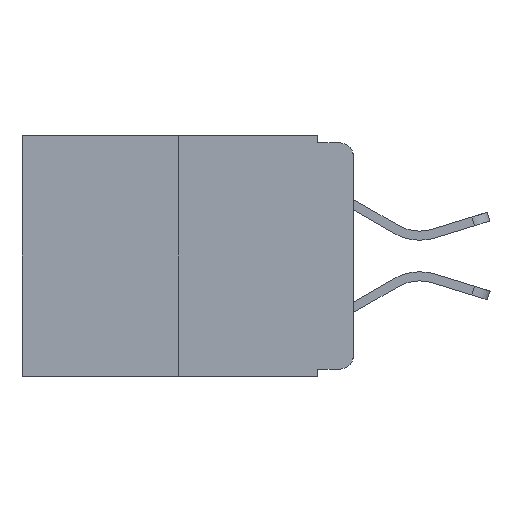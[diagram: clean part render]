
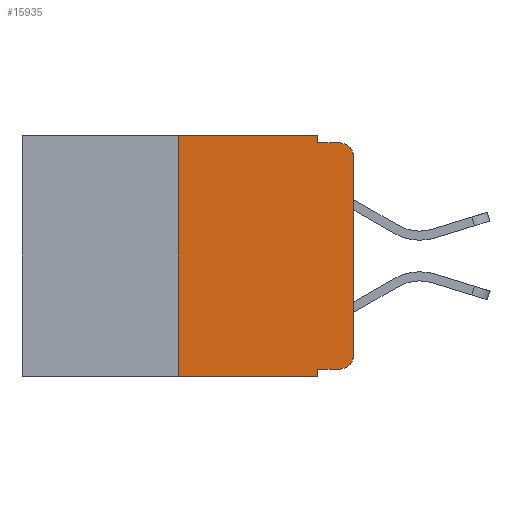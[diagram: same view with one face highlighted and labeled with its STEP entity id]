
A CAD part, left-side view. The second image highlights one B-rep face of the part: STEP entity #15935.
In plain terms, the highlighted planar face has unit normal (-1, 0, 0).
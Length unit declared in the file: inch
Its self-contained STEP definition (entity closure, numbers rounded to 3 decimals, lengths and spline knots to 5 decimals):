
#294 = CARTESIAN_POINT ( 'NONE',  ( 0., 0.051, -0.333 ) ) ;
#400 = VECTOR ( 'NONE', #10539, 39.37008 ) ;
#865 = EDGE_CURVE ( 'NONE', #15605, #11116, #6117, .T. ) ;
#1039 = LINE ( 'NONE', #8355, #7173 ) ;
#1215 = DIRECTION ( 'NONE',  ( 0., 0., 1. ) ) ;
#1316 = AXIS2_PLACEMENT_3D ( 'NONE', #6668, #11313, #2553 ) ;
#1651 = VERTEX_POINT ( 'NONE', #7602 ) ;
#1669 = CARTESIAN_POINT ( 'NONE',  ( 0., 0.25, 0. ) ) ;
#2003 = ORIENTED_EDGE ( 'NONE', *, *, #8652, .F. ) ;
#2007 = CARTESIAN_POINT ( 'NONE',  ( 0., 0.02, -0.03 ) ) ;
#2306 = DIRECTION ( 'NONE',  ( 0., -1., 0. ) ) ;
#2553 = DIRECTION ( 'NONE',  ( 0., 0., -1. ) ) ;
#2611 = EDGE_CURVE ( 'NONE', #11900, #15605, #6911, .T. ) ;
#2836 = LINE ( 'NONE', #11430, #16879 ) ;
#3022 = CARTESIAN_POINT ( 'NONE',  ( 0., 0., 0. ) ) ;
#3719 = ORIENTED_EDGE ( 'NONE', *, *, #9662, .F. ) ;
#4295 = DIRECTION ( 'NONE',  ( 0., -1., 0. ) ) ;
#4347 = EDGE_CURVE ( 'NONE', #10355, #1651, #14121, .T. ) ;
#4500 = VECTOR ( 'NONE', #1215, 39.37008 ) ;
#4568 = LINE ( 'NONE', #8996, #400 ) ;
#5197 = DIRECTION ( 'NONE',  ( 0., 0., 1. ) ) ;
#5552 = DIRECTION ( 'NONE',  ( 0., 0., -1. ) ) ;
#5730 = LINE ( 'NONE', #17534, #10146 ) ;
#5777 = EDGE_CURVE ( 'NONE', #10741, #11241, #5730, .T. ) ;
#6117 = CIRCLE ( 'NONE', #16936, 0.02 ) ;
#6533 = EDGE_CURVE ( 'NONE', #15993, #1651, #16504, .T. ) ;
#6590 = CARTESIAN_POINT ( 'NONE',  ( 0., 0.02, -0.313 ) ) ;
#6668 = CARTESIAN_POINT ( 'NONE',  ( 0., 0.473, 0. ) ) ;
#6734 = LINE ( 'NONE', #15803, #13679 ) ;
#6768 = PLANE ( 'NONE',  #1316 ) ;
#6911 = LINE ( 'NONE', #17268, #8942 ) ;
#7173 = VECTOR ( 'NONE', #2306, 39.37008 ) ;
#7587 = ORIENTED_EDGE ( 'NONE', *, *, #16901, .F. ) ;
#7602 = CARTESIAN_POINT ( 'NONE',  ( 0., 0.02, -0.01 ) ) ;
#7891 = EDGE_CURVE ( 'NONE', #18049, #15824, #1039, .T. ) ;
#8130 = CARTESIAN_POINT ( 'NONE',  ( 0., 0.051, -0.343 ) ) ;
#8355 = CARTESIAN_POINT ( 'NONE',  ( 0., 0.473, -0.343 ) ) ;
#8652 = EDGE_CURVE ( 'NONE', #18049, #10741, #6734, .T. ) ;
#8942 = VECTOR ( 'NONE', #12995, 39.37008 ) ;
#8996 = CARTESIAN_POINT ( 'NONE',  ( 0., 0.051, 0. ) ) ;
#9662 = EDGE_CURVE ( 'NONE', #11900, #15824, #2836, .T. ) ;
#9881 = ORIENTED_EDGE ( 'NONE', *, *, #7891, .T. ) ;
#9899 = ORIENTED_EDGE ( 'NONE', *, *, #2611, .T. ) ;
#9979 = CARTESIAN_POINT ( 'NONE',  ( 0., 0.25, -0.343 ) ) ;
#10015 = ORIENTED_EDGE ( 'NONE', *, *, #6533, .F. ) ;
#10146 = VECTOR ( 'NONE', #4295, 39.37008 ) ;
#10355 = VERTEX_POINT ( 'NONE', #18428 ) ;
#10539 = DIRECTION ( 'NONE',  ( 0., 0., -1. ) ) ;
#10741 = VERTEX_POINT ( 'NONE', #1669 ) ;
#11116 = VERTEX_POINT ( 'NONE', #18305 ) ;
#11241 = VERTEX_POINT ( 'NONE', #16039 ) ;
#11313 = DIRECTION ( 'NONE',  ( 1., 0., 0. ) ) ;
#11430 = CARTESIAN_POINT ( 'NONE',  ( 0., 0.051, 0. ) ) ;
#11527 = LINE ( 'NONE', #3022, #4500 ) ;
#11900 = VERTEX_POINT ( 'NONE', #294 ) ;
#12059 = CARTESIAN_POINT ( 'NONE',  ( 0., 0.051, -0.01 ) ) ;
#12681 = DIRECTION ( 'NONE',  ( -1., 0., 0. ) ) ;
#12700 = EDGE_CURVE ( 'NONE', #11116, #10355, #11527, .T. ) ;
#12995 = DIRECTION ( 'NONE',  ( 0., -1., 0. ) ) ;
#13608 = CARTESIAN_POINT ( 'NONE',  ( 0., 0.051, -0.01 ) ) ;
#13679 = VECTOR ( 'NONE', #5197, 39.37008 ) ;
#13752 = DIRECTION ( 'NONE',  ( -1., 0., 0. ) ) ;
#14121 = CIRCLE ( 'NONE', #15668, 0.02 ) ;
#14202 = ORIENTED_EDGE ( 'NONE', *, *, #12700, .T. ) ;
#14303 = DIRECTION ( 'NONE',  ( 0., 0., -1. ) ) ;
#14853 = ORIENTED_EDGE ( 'NONE', *, *, #865, .T. ) ;
#15357 = DIRECTION ( 'NONE',  ( 0., -1., 0. ) ) ;
#15461 = VECTOR ( 'NONE', #15357, 39.37008 ) ;
#15605 = VERTEX_POINT ( 'NONE', #15766 ) ;
#15668 = AXIS2_PLACEMENT_3D ( 'NONE', #2007, #13752, #5552 ) ;
#15766 = CARTESIAN_POINT ( 'NONE',  ( 0., 0.02, -0.333 ) ) ;
#15803 = CARTESIAN_POINT ( 'NONE',  ( 0., 0.25, 0. ) ) ;
#15824 = VERTEX_POINT ( 'NONE', #8130 ) ;
#15838 = FACE_OUTER_BOUND ( 'NONE', #17122, .T. ) ;
#15935 = ADVANCED_FACE ( 'NONE', ( #15838 ), #6768, .F. ) ;
#15993 = VERTEX_POINT ( 'NONE', #12059 ) ;
#16039 = CARTESIAN_POINT ( 'NONE',  ( 0., 0.051, 0. ) ) ;
#16139 = ORIENTED_EDGE ( 'NONE', *, *, #5777, .F. ) ;
#16504 = LINE ( 'NONE', #13608, #15461 ) ;
#16879 = VECTOR ( 'NONE', #17322, 39.37008 ) ;
#16901 = EDGE_CURVE ( 'NONE', #11241, #15993, #4568, .T. ) ;
#16924 = ORIENTED_EDGE ( 'NONE', *, *, #4347, .T. ) ;
#16936 = AXIS2_PLACEMENT_3D ( 'NONE', #6590, #12681, #14303 ) ;
#17122 = EDGE_LOOP ( 'NONE', ( #14202, #16924, #10015, #7587, #16139, #2003, #9881, #3719, #9899, #14853 ) ) ;
#17268 = CARTESIAN_POINT ( 'NONE',  ( 0., 0.051, -0.333 ) ) ;
#17322 = DIRECTION ( 'NONE',  ( 0., 0., -1. ) ) ;
#17534 = CARTESIAN_POINT ( 'NONE',  ( 0., 0.473, 0. ) ) ;
#18049 = VERTEX_POINT ( 'NONE', #9979 ) ;
#18305 = CARTESIAN_POINT ( 'NONE',  ( 0., 0., -0.313 ) ) ;
#18428 = CARTESIAN_POINT ( 'NONE',  ( 0., 0., -0.03 ) ) ;
